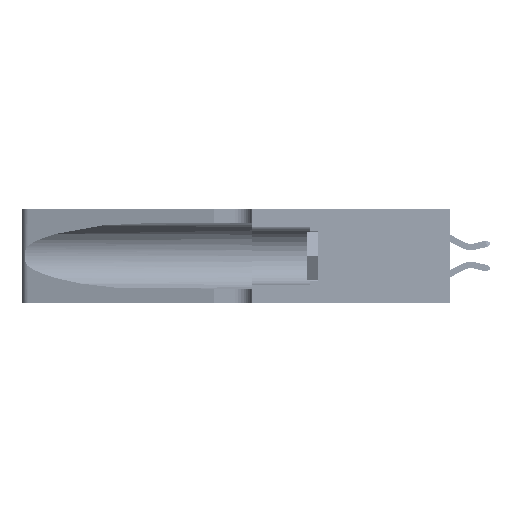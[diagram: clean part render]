
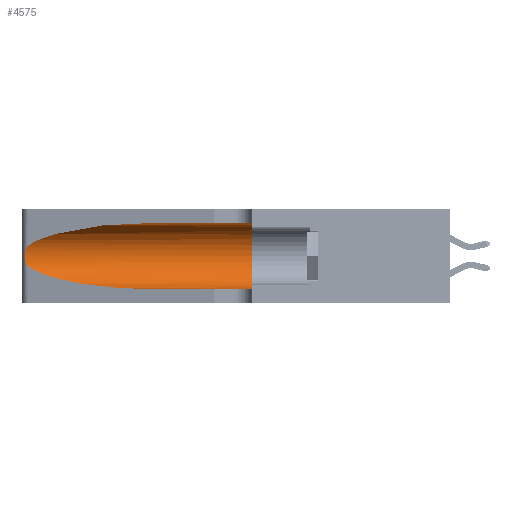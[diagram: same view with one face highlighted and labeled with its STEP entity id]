
A CAD part, left-side view. The second image highlights one B-rep face of the part: STEP entity #4575.
In plain terms, the highlighted cylindrical face has radius 3.308 mm (diameter 6.617 mm), a partial arc.
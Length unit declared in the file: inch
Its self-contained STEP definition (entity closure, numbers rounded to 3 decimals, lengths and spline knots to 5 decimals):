
#202 = DIRECTION ( 'NONE',  ( 0., -1., 0. ) ) ;
#769 = ORIENTED_EDGE ( 'NONE', *, *, #6257, .F. ) ;
#1606 = CIRCLE ( 'NONE', #16950, 0.13025 ) ;
#1681 = VERTEX_POINT ( 'NONE', #40273 ) ;
#2055 = CARTESIAN_POINT ( 'NONE',  ( 0.25856, 1.23593, 0.16098 ) ) ;
#2246 = CARTESIAN_POINT ( 'NONE',  ( 0.25487, 1.22718, 0.14631 ) ) ;
#4153 = ORIENTED_EDGE ( 'NONE', *, *, #11226, .T. ) ;
#4292 = ORIENTED_EDGE ( 'NONE', *, *, #7094, .F. ) ;
#4479 = CARTESIAN_POINT ( 'NONE',  ( 0.25487, 1.22718, 0.22369 ) ) ;
#4575 = ADVANCED_FACE ( 'NONE', ( #13887 ), #32403, .F. ) ;
#5653 = CARTESIAN_POINT ( 'NONE',  ( 0.25555, 1.22994, 0.2215 ) ) ;
#5811 = CARTESIAN_POINT ( 'NONE',  ( 0.25639, 1.23186, 0.15144 ) ) ;
#6257 = EDGE_CURVE ( 'NONE', #1681, #36948, #1606, .T. ) ;
#6582 = ORIENTED_EDGE ( 'NONE', *, *, #18118, .T. ) ;
#6722 = CARTESIAN_POINT ( 'NONE',  ( 0.1305, 0.72297, 0.31525 ) ) ;
#6777 = CARTESIAN_POINT ( 'NONE',  ( 0.1305, 0.35, 0.185 ) ) ;
#7094 = EDGE_CURVE ( 'NONE', #47181, #1681, #33550, .T. ) ;
#9541 = CARTESIAN_POINT ( 'NONE',  ( 0.25487, 1.22718, 0.14631 ) ) ;
#9738 = CARTESIAN_POINT ( 'NONE',  ( 0.18966, 0.96281, 0.05475 ) ) ;
#10532 = DIRECTION ( 'NONE',  ( 0., 0., 1. ) ) ;
#11226 = EDGE_CURVE ( 'NONE', #22297, #17319, #27665, .T. ) ;
#13100 = CARTESIAN_POINT ( 'NONE',  ( 0.25487, 1.22718, 0.22369 ) ) ;
#13887 = FACE_OUTER_BOUND ( 'NONE', #47150, .T. ) ;
#15187 = CARTESIAN_POINT ( 'NONE',  ( 0.1305, 1.61858, 0.185 ) ) ;
#16836 = CARTESIAN_POINT ( 'NONE',  ( 0.25854, 1.2359, 0.20912 ) ) ;
#16950 = AXIS2_PLACEMENT_3D ( 'NONE', #6777, #32667, #10532 ) ;
#17319 = VERTEX_POINT ( 'NONE', #31297 ) ;
#18118 = EDGE_CURVE ( 'NONE', #17319, #35598, #19096, .T. ) ;
#18169 = CARTESIAN_POINT ( 'NONE',  ( 0.2373, 1.15595, 0.28018 ) ) ;
#18501 = AXIS2_PLACEMENT_3D ( 'NONE', #15187, #29906, #40997 ) ;
#19096 =( BOUNDED_CURVE ( )  B_SPLINE_CURVE ( 3, ( #2246, #31879, #9738, #35576 ),
 .UNSPECIFIED., .F., .F. ) 
 B_SPLINE_CURVE_WITH_KNOTS ( ( 4, 4 ),
 ( 3.44316, 4.71239 ),
 .UNSPECIFIED. ) 
 CURVE ( )  GEOMETRIC_REPRESENTATION_ITEM ( )  RATIONAL_B_SPLINE_CURVE ( ( 1., 0.87, 0.87, 1. ) ) 
 REPRESENTATION_ITEM ( '' )  );
#19445 = DIRECTION ( 'NONE',  ( 0., -1., 0. ) ) ;
#20578 = CARTESIAN_POINT ( 'NONE',  ( 0.26075, 1.23896, 0.19203 ) ) ;
#22297 = VERTEX_POINT ( 'NONE', #4479 ) ;
#24274 = CARTESIAN_POINT ( 'NONE',  ( 0.26017, 1.23833, 0.17102 ) ) ;
#24543 = CARTESIAN_POINT ( 'NONE',  ( 0.1305, 0.35, 0.05475 ) ) ;
#27665 = B_SPLINE_CURVE_WITH_KNOTS ( 'NONE', 3,
 ( #13100, #5653, #27826, #38931, #16836, #42625, #20578, #46293, #24274, #2055, #27986, #5811, #31686, #9541 ),
 .UNSPECIFIED., .F., .F.,
 ( 4, 2, 2, 2, 2, 2, 4 ),
 ( 0., 0.00027, 0.00053, 0.00107, 0.0016, 0.00187, 0.00214 ),
 .UNSPECIFIED. ) ;
#27826 = CARTESIAN_POINT ( 'NONE',  ( 0.25639, 1.23184, 0.21858 ) ) ;
#27986 = CARTESIAN_POINT ( 'NONE',  ( 0.25789, 1.23486, 0.15765 ) ) ;
#28686 = CARTESIAN_POINT ( 'NONE',  ( 0.1305, 0.72297, 0.05475 ) ) ;
#29906 = DIRECTION ( 'NONE',  ( 0., -1., 0. ) ) ;
#31297 = CARTESIAN_POINT ( 'NONE',  ( 0.25487, 1.22718, 0.14631 ) ) ;
#31686 = CARTESIAN_POINT ( 'NONE',  ( 0.25555, 1.22993, 0.14849 ) ) ;
#31879 = CARTESIAN_POINT ( 'NONE',  ( 0.2373, 1.15595, 0.08982 ) ) ;
#32395 = ORIENTED_EDGE ( 'NONE', *, *, #41329, .T. ) ;
#32403 = CYLINDRICAL_SURFACE ( 'NONE', #18501, 0.13025 ) ;
#32667 = DIRECTION ( 'NONE',  ( 0., 1., 0. ) ) ;
#33550 = LINE ( 'NONE', #44474, #42172 ) ;
#33952 = CARTESIAN_POINT ( 'NONE',  ( 0.1305, 1.61858, 0.05475 ) ) ;
#34647 = EDGE_CURVE ( 'NONE', #35598, #36948, #46709, .T. ) ;
#35576 = CARTESIAN_POINT ( 'NONE',  ( 0.1305, 0.72297, 0.05475 ) ) ;
#35598 = VERTEX_POINT ( 'NONE', #28686 ) ;
#35813 = VECTOR ( 'NONE', #19445, 39.37008 ) ;
#36548 = CARTESIAN_POINT ( 'NONE',  ( 0.18966, 0.96281, 0.31525 ) ) ;
#36948 = VERTEX_POINT ( 'NONE', #24543 ) ;
#37695 =( BOUNDED_CURVE ( )  B_SPLINE_CURVE ( 3, ( #40076, #36548, #18169, #43917 ),
 .UNSPECIFIED., .F., .F. ) 
 B_SPLINE_CURVE_WITH_KNOTS ( ( 4, 4 ),
 ( 1.5708, 2.84003 ),
 .UNSPECIFIED. ) 
 CURVE ( )  GEOMETRIC_REPRESENTATION_ITEM ( )  RATIONAL_B_SPLINE_CURVE ( ( 1., 0.87, 0.87, 1. ) ) 
 REPRESENTATION_ITEM ( '' )  );
#38931 = CARTESIAN_POINT ( 'NONE',  ( 0.25787, 1.23484, 0.2124 ) ) ;
#39539 = ORIENTED_EDGE ( 'NONE', *, *, #34647, .T. ) ;
#40076 = CARTESIAN_POINT ( 'NONE',  ( 0.1305, 0.72297, 0.31525 ) ) ;
#40273 = CARTESIAN_POINT ( 'NONE',  ( 0.1305, 0.35, 0.31525 ) ) ;
#40997 = DIRECTION ( 'NONE',  ( 0., 0., -1. ) ) ;
#41329 = EDGE_CURVE ( 'NONE', #47181, #22297, #37695, .T. ) ;
#42172 = VECTOR ( 'NONE', #202, 39.37008 ) ;
#42625 = CARTESIAN_POINT ( 'NONE',  ( 0.26018, 1.23835, 0.19895 ) ) ;
#43917 = CARTESIAN_POINT ( 'NONE',  ( 0.25487, 1.22718, 0.22369 ) ) ;
#44474 = CARTESIAN_POINT ( 'NONE',  ( 0.1305, 1.61858, 0.31525 ) ) ;
#46293 = CARTESIAN_POINT ( 'NONE',  ( 0.26075, 1.23896, 0.178 ) ) ;
#46709 = LINE ( 'NONE', #33952, #35813 ) ;
#47150 = EDGE_LOOP ( 'NONE', ( #32395, #4153, #6582, #39539, #769, #4292 ) ) ;
#47181 = VERTEX_POINT ( 'NONE', #6722 ) ;
